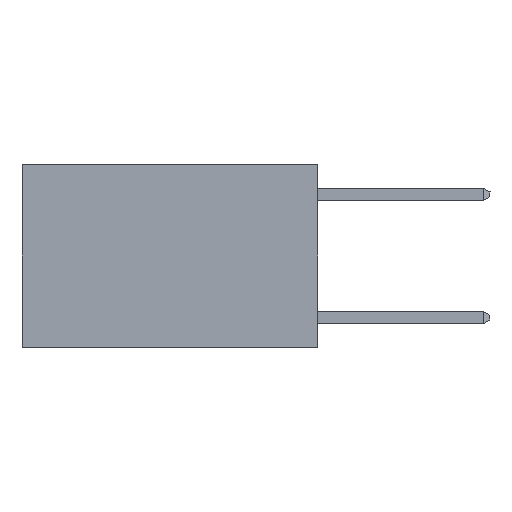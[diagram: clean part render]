
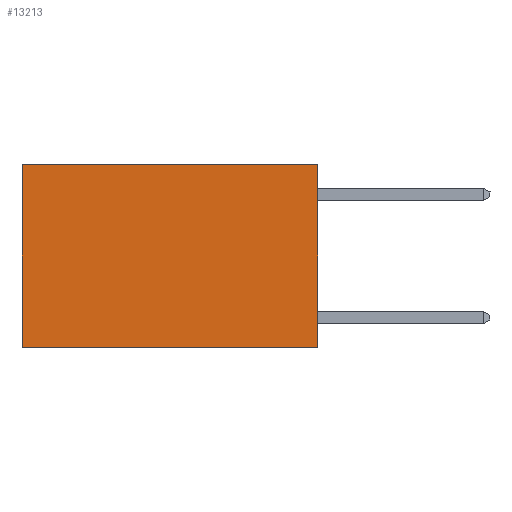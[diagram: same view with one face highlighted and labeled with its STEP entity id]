
A CAD part, left-side view. The second image highlights one B-rep face of the part: STEP entity #13213.
In plain terms, the highlighted planar face has unit normal (-1, 0, 0).
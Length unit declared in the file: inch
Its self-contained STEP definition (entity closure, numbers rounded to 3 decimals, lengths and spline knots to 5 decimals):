
#45 = CARTESIAN_POINT ( 'NONE',  ( 0.2625, 0.6, 0. ) ) ;
#718 = LINE ( 'NONE', #9537, #10343 ) ;
#923 = EDGE_LOOP ( 'NONE', ( #13924, #12634, #10857, #8258 ) ) ;
#1035 = VECTOR ( 'NONE', #3252, 39.37008 ) ;
#1749 = EDGE_CURVE ( 'NONE', #14568, #12065, #718, .T. ) ;
#3252 = DIRECTION ( 'NONE',  ( 0., 0., -1. ) ) ;
#3610 = EDGE_CURVE ( 'NONE', #12065, #5024, #4770, .T. ) ;
#4328 = EDGE_CURVE ( 'NONE', #5965, #5024, #14214, .T. ) ;
#4770 = LINE ( 'NONE', #14596, #1035 ) ;
#5024 = VERTEX_POINT ( 'NONE', #14939 ) ;
#5393 = VECTOR ( 'NONE', #6907, 39.37008 ) ;
#5637 = CARTESIAN_POINT ( 'NONE',  ( 0.2625, 0., 0. ) ) ;
#5785 = LINE ( 'NONE', #5637, #5393 ) ;
#5828 = DIRECTION ( 'NONE',  ( 1., 0., 0. ) ) ;
#5965 = VERTEX_POINT ( 'NONE', #12359 ) ;
#6312 = CARTESIAN_POINT ( 'NONE',  ( 0.2625, 0., 0. ) ) ;
#6907 = DIRECTION ( 'NONE',  ( 0., 0., -1. ) ) ;
#7112 = EDGE_CURVE ( 'NONE', #14568, #5965, #5785, .T. ) ;
#8258 = ORIENTED_EDGE ( 'NONE', *, *, #1749, .T. ) ;
#9537 = CARTESIAN_POINT ( 'NONE',  ( 0.2625, 0., 0. ) ) ;
#9577 = CARTESIAN_POINT ( 'NONE',  ( 0.2625, 0., 0. ) ) ;
#9730 = DIRECTION ( 'NONE',  ( 0., 1., 0. ) ) ;
#10343 = VECTOR ( 'NONE', #9730, 39.37008 ) ;
#10857 = ORIENTED_EDGE ( 'NONE', *, *, #7112, .F. ) ;
#11667 = AXIS2_PLACEMENT_3D ( 'NONE', #9577, #5828, #14651 ) ;
#12065 = VERTEX_POINT ( 'NONE', #45 ) ;
#12359 = CARTESIAN_POINT ( 'NONE',  ( 0.2625, 0., -0.37 ) ) ;
#12634 = ORIENTED_EDGE ( 'NONE', *, *, #4328, .F. ) ;
#13213 = ADVANCED_FACE ( 'NONE', ( #15623 ), #13401, .F. ) ;
#13401 = PLANE ( 'NONE',  #11667 ) ;
#13600 = CARTESIAN_POINT ( 'NONE',  ( 0.2625, 0., -0.37 ) ) ;
#13828 = VECTOR ( 'NONE', #14796, 39.37008 ) ;
#13924 = ORIENTED_EDGE ( 'NONE', *, *, #3610, .T. ) ;
#14214 = LINE ( 'NONE', #13600, #13828 ) ;
#14568 = VERTEX_POINT ( 'NONE', #6312 ) ;
#14596 = CARTESIAN_POINT ( 'NONE',  ( 0.2625, 0.6, 0. ) ) ;
#14651 = DIRECTION ( 'NONE',  ( 0., 0., -1. ) ) ;
#14796 = DIRECTION ( 'NONE',  ( 0., 1., 0. ) ) ;
#14939 = CARTESIAN_POINT ( 'NONE',  ( 0.2625, 0.6, -0.37 ) ) ;
#15623 = FACE_OUTER_BOUND ( 'NONE', #923, .T. ) ;
